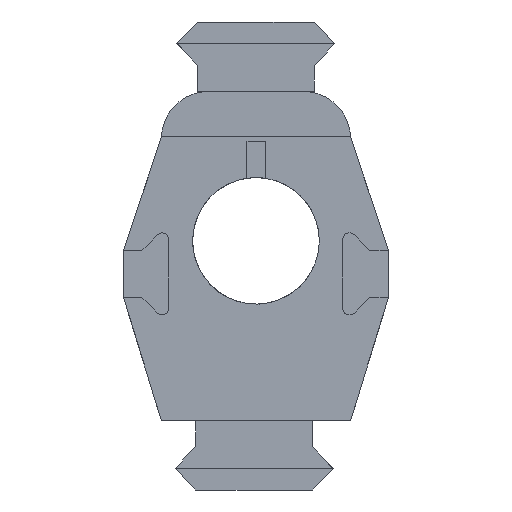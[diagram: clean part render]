
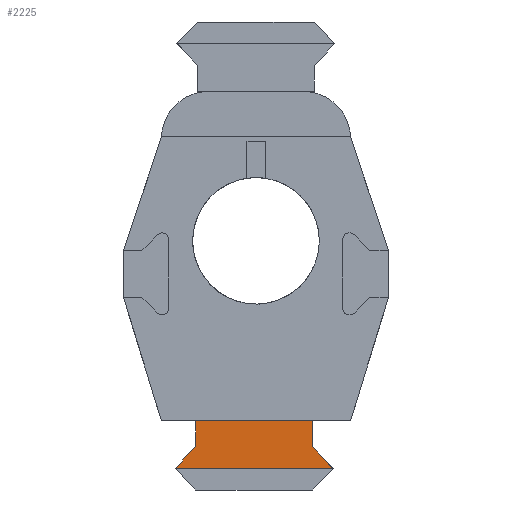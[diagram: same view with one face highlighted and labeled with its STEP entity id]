
A CAD part, front view. The second image highlights one B-rep face of the part: STEP entity #2225.
In plain terms, the highlighted planar face has unit normal (0, -1, 0).
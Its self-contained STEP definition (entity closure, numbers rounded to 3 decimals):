
#162=FACE_OUTER_BOUND('',#287,.T.);
#287=EDGE_LOOP('',(#1783,#1784,#1785,#1786,#1787,#1788));
#466=LINE('',#3452,#740);
#484=LINE('',#3487,#758);
#487=LINE('',#3493,#761);
#488=LINE('',#3496,#762);
#489=LINE('',#3498,#763);
#490=LINE('',#3499,#764);
#740=VECTOR('',#2800,10.);
#758=VECTOR('',#2820,10.);
#761=VECTOR('',#2825,10.);
#762=VECTOR('',#2828,10.);
#763=VECTOR('',#2829,10.);
#764=VECTOR('',#2830,10.);
#1003=VERTEX_POINT('',#3449);
#1004=VERTEX_POINT('',#3451);
#1020=VERTEX_POINT('',#3485);
#1022=VERTEX_POINT('',#3491);
#1023=VERTEX_POINT('',#3495);
#1024=VERTEX_POINT('',#3497);
#1269=EDGE_CURVE('',#1003,#1004,#466,.T.);
#1287=EDGE_CURVE('',#1020,#1003,#484,.T.);
#1290=EDGE_CURVE('',#1022,#1020,#487,.T.);
#1291=EDGE_CURVE('',#1023,#1022,#488,.T.);
#1292=EDGE_CURVE('',#1024,#1023,#489,.T.);
#1293=EDGE_CURVE('',#1004,#1024,#490,.T.);
#1783=ORIENTED_EDGE('',*,*,#1287,.F.);
#1784=ORIENTED_EDGE('',*,*,#1290,.F.);
#1785=ORIENTED_EDGE('',*,*,#1291,.F.);
#1786=ORIENTED_EDGE('',*,*,#1292,.F.);
#1787=ORIENTED_EDGE('',*,*,#1293,.F.);
#1788=ORIENTED_EDGE('',*,*,#1269,.F.);
#2104=PLANE('',#2407);
#2225=ADVANCED_FACE('',(#162),#2104,.F.);
#2407=AXIS2_PLACEMENT_3D('',#3494,#2826,#2827);
#2800=DIRECTION('',(0.691,0.,-0.723));
#2820=DIRECTION('',(0.,0.,-1.));
#2825=DIRECTION('',(1.,0.,0.));
#2826=DIRECTION('center_axis',(0.,1.,0.));
#2827=DIRECTION('ref_axis',(0.,0.,1.));
#2828=DIRECTION('',(0.,0.,1.));
#2829=DIRECTION('',(0.689,0.,0.725));
#2830=DIRECTION('',(-1.,0.,0.));
#3449=CARTESIAN_POINT('',(7.582,171.04,-16.235));
#3451=CARTESIAN_POINT('',(10.321,171.04,-19.102));
#3452=CARTESIAN_POINT('',(6.671,171.04,-15.282));
#3485=CARTESIAN_POINT('',(7.582,171.04,-12.7));
#3487=CARTESIAN_POINT('',(7.582,171.04,-19.129));
#3491=CARTESIAN_POINT('',(-8.09,171.04,-12.7));
#3493=CARTESIAN_POINT('',(-0.254,171.04,-12.7));
#3494=CARTESIAN_POINT('Origin',(-8.09,171.04,-22.022));
#3495=CARTESIAN_POINT('',(-8.09,171.04,-16.19));
#3496=CARTESIAN_POINT('',(-8.09,171.04,-17.361));
#3497=CARTESIAN_POINT('',(-10.858,171.04,-19.102));
#3498=CARTESIAN_POINT('',(-9.546,171.04,-17.721));
#3499=CARTESIAN_POINT('',(-8.09,171.04,-19.102));
